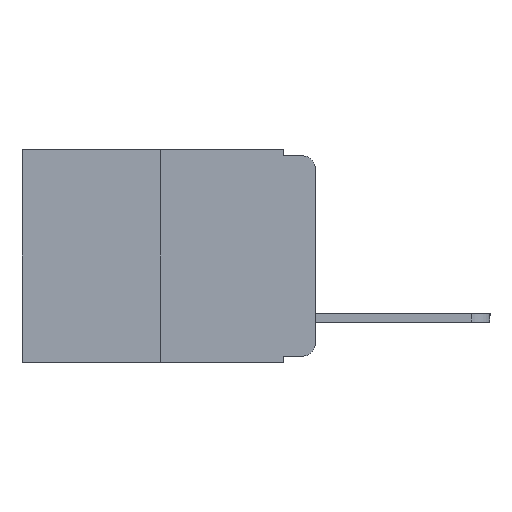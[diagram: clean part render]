
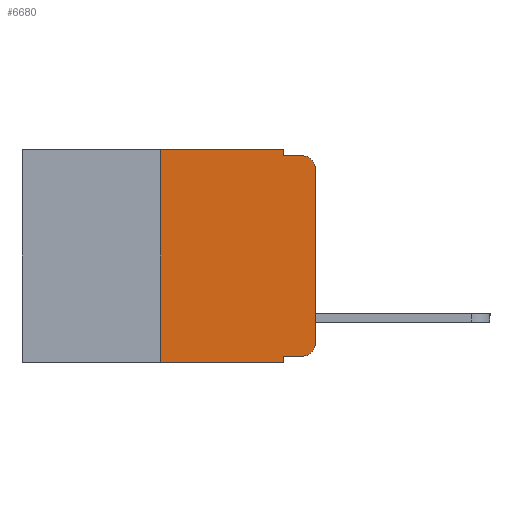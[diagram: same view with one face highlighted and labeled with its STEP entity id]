
A CAD part, left-side view. The second image highlights one B-rep face of the part: STEP entity #6680.
In plain terms, the highlighted planar face has unit normal (-1, 0, 0).
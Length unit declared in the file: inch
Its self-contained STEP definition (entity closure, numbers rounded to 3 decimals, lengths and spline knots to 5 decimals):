
#320 = CARTESIAN_POINT ( 'NONE',  ( 0., 0.051, 0. ) ) ;
#336 = EDGE_CURVE ( 'NONE', #5098, #11515, #13873, .T. ) ;
#733 = CARTESIAN_POINT ( 'NONE',  ( 0., 0.051, -0.333 ) ) ;
#815 = DIRECTION ( 'NONE',  ( 0., 0., 1. ) ) ;
#819 = VECTOR ( 'NONE', #1207, 39.37008 ) ;
#828 = EDGE_CURVE ( 'NONE', #10019, #2512, #13077, .T. ) ;
#859 = EDGE_CURVE ( 'NONE', #15618, #13723, #9043, .T. ) ;
#1207 = DIRECTION ( 'NONE',  ( 0., -1., 0. ) ) ;
#1308 = CARTESIAN_POINT ( 'NONE',  ( 0., 0.051, -0.343 ) ) ;
#1365 = DIRECTION ( 'NONE',  ( 0., 0., -1. ) ) ;
#1665 = VECTOR ( 'NONE', #1365, 39.37008 ) ;
#2113 = LINE ( 'NONE', #320, #1665 ) ;
#2512 = VERTEX_POINT ( 'NONE', #6368 ) ;
#2865 = ORIENTED_EDGE ( 'NONE', *, *, #10390, .T. ) ;
#3595 = ORIENTED_EDGE ( 'NONE', *, *, #7487, .F. ) ;
#3763 = CARTESIAN_POINT ( 'NONE',  ( 0., 0.473, 0. ) ) ;
#4743 = VECTOR ( 'NONE', #815, 39.37008 ) ;
#4761 = EDGE_CURVE ( 'NONE', #13734, #10019, #14072, .T. ) ;
#4959 = CARTESIAN_POINT ( 'NONE',  ( 0., 0.02, -0.01 ) ) ;
#5046 = CARTESIAN_POINT ( 'NONE',  ( 0., 0.02, -0.03 ) ) ;
#5098 = VERTEX_POINT ( 'NONE', #15868 ) ;
#5157 = CARTESIAN_POINT ( 'NONE',  ( 0., 0.051, 0. ) ) ;
#5465 = AXIS2_PLACEMENT_3D ( 'NONE', #7515, #6499, #6125 ) ;
#5486 = ORIENTED_EDGE ( 'NONE', *, *, #9639, .F. ) ;
#5526 = VERTEX_POINT ( 'NONE', #12174 ) ;
#5554 = CARTESIAN_POINT ( 'NONE',  ( 0., 0.25, 0. ) ) ;
#5654 = VECTOR ( 'NONE', #9503, 39.37008 ) ;
#5704 = EDGE_LOOP ( 'NONE', ( #9873, #2865, #13491, #5486, #16131, #15581, #15782, #3595, #11250, #11068 ) ) ;
#5716 = CARTESIAN_POINT ( 'NONE',  ( 0., 0.473, -0.343 ) ) ;
#6125 = DIRECTION ( 'NONE',  ( 0., 0., -1. ) ) ;
#6368 = CARTESIAN_POINT ( 'NONE',  ( 0., 0., -0.313 ) ) ;
#6436 = DIRECTION ( 'NONE',  ( 0., -1., 0. ) ) ;
#6499 = DIRECTION ( 'NONE',  ( 1., 0., 0. ) ) ;
#6680 = ADVANCED_FACE ( 'NONE', ( #14419 ), #10060, .F. ) ;
#6747 = AXIS2_PLACEMENT_3D ( 'NONE', #14370, #12946, #14346 ) ;
#6852 = VECTOR ( 'NONE', #14726, 39.37008 ) ;
#6895 = DIRECTION ( 'NONE',  ( 0., 0., 1. ) ) ;
#7229 = LINE ( 'NONE', #5157, #6852 ) ;
#7358 = DIRECTION ( 'NONE',  ( -1., 0., 0. ) ) ;
#7413 = DIRECTION ( 'NONE',  ( 0., 0., -1. ) ) ;
#7487 = EDGE_CURVE ( 'NONE', #13734, #11515, #2113, .T. ) ;
#7515 = CARTESIAN_POINT ( 'NONE',  ( 0., 0.473, 0. ) ) ;
#7875 = CARTESIAN_POINT ( 'NONE',  ( 0., 0., -0.03 ) ) ;
#8569 = LINE ( 'NONE', #5554, #11442 ) ;
#8972 = CARTESIAN_POINT ( 'NONE',  ( 0., 0.051, -0.01 ) ) ;
#9043 = LINE ( 'NONE', #8972, #5654 ) ;
#9203 = LINE ( 'NONE', #3763, #12089 ) ;
#9503 = DIRECTION ( 'NONE',  ( 0., -1., 0. ) ) ;
#9639 = EDGE_CURVE ( 'NONE', #12325, #15618, #7229, .T. ) ;
#9753 = EDGE_CURVE ( 'NONE', #2512, #11841, #9770, .T. ) ;
#9770 = LINE ( 'NONE', #13992, #4743 ) ;
#9814 = CARTESIAN_POINT ( 'NONE',  ( 0., 0.051, 0. ) ) ;
#9873 = ORIENTED_EDGE ( 'NONE', *, *, #9753, .T. ) ;
#10019 = VERTEX_POINT ( 'NONE', #14270 ) ;
#10060 = PLANE ( 'NONE',  #5465 ) ;
#10147 = CIRCLE ( 'NONE', #11600, 0.02 ) ;
#10390 = EDGE_CURVE ( 'NONE', #11841, #13723, #10147, .T. ) ;
#10829 = VECTOR ( 'NONE', #6436, 39.37008 ) ;
#11068 = ORIENTED_EDGE ( 'NONE', *, *, #828, .T. ) ;
#11250 = ORIENTED_EDGE ( 'NONE', *, *, #4761, .T. ) ;
#11442 = VECTOR ( 'NONE', #6895, 39.37008 ) ;
#11492 = EDGE_CURVE ( 'NONE', #5098, #5526, #8569, .T. ) ;
#11515 = VERTEX_POINT ( 'NONE', #1308 ) ;
#11600 = AXIS2_PLACEMENT_3D ( 'NONE', #5046, #7358, #7413 ) ;
#11841 = VERTEX_POINT ( 'NONE', #7875 ) ;
#11996 = CARTESIAN_POINT ( 'NONE',  ( 0., 0.051, -0.01 ) ) ;
#12089 = VECTOR ( 'NONE', #13921, 39.37008 ) ;
#12174 = CARTESIAN_POINT ( 'NONE',  ( 0., 0.25, 0. ) ) ;
#12325 = VERTEX_POINT ( 'NONE', #9814 ) ;
#12946 = DIRECTION ( 'NONE',  ( -1., 0., 0. ) ) ;
#13077 = CIRCLE ( 'NONE', #6747, 0.02 ) ;
#13491 = ORIENTED_EDGE ( 'NONE', *, *, #859, .F. ) ;
#13723 = VERTEX_POINT ( 'NONE', #4959 ) ;
#13734 = VERTEX_POINT ( 'NONE', #733 ) ;
#13873 = LINE ( 'NONE', #5716, #819 ) ;
#13921 = DIRECTION ( 'NONE',  ( 0., -1., 0. ) ) ;
#13992 = CARTESIAN_POINT ( 'NONE',  ( 0., 0., 0. ) ) ;
#14072 = LINE ( 'NONE', #16046, #10829 ) ;
#14270 = CARTESIAN_POINT ( 'NONE',  ( 0., 0.02, -0.333 ) ) ;
#14346 = DIRECTION ( 'NONE',  ( 0., 0., -1. ) ) ;
#14370 = CARTESIAN_POINT ( 'NONE',  ( 0., 0.02, -0.313 ) ) ;
#14419 = FACE_OUTER_BOUND ( 'NONE', #5704, .T. ) ;
#14726 = DIRECTION ( 'NONE',  ( 0., 0., -1. ) ) ;
#15581 = ORIENTED_EDGE ( 'NONE', *, *, #11492, .F. ) ;
#15618 = VERTEX_POINT ( 'NONE', #11996 ) ;
#15782 = ORIENTED_EDGE ( 'NONE', *, *, #336, .T. ) ;
#15868 = CARTESIAN_POINT ( 'NONE',  ( 0., 0.25, -0.343 ) ) ;
#16046 = CARTESIAN_POINT ( 'NONE',  ( 0., 0.051, -0.333 ) ) ;
#16131 = ORIENTED_EDGE ( 'NONE', *, *, #16635, .F. ) ;
#16635 = EDGE_CURVE ( 'NONE', #5526, #12325, #9203, .T. ) ;
